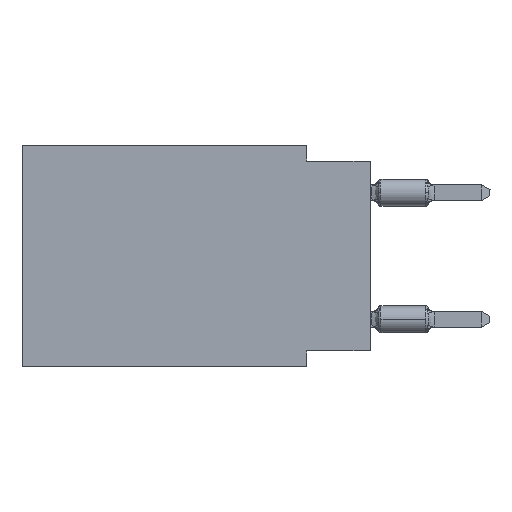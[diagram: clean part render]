
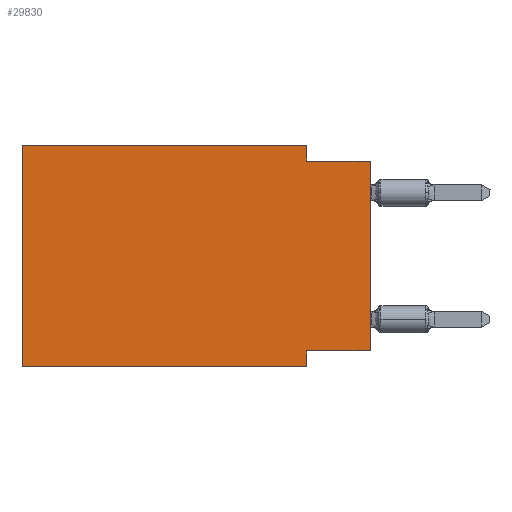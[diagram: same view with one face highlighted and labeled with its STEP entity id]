
A CAD part, left-side view. The second image highlights one B-rep face of the part: STEP entity #29830.
In plain terms, the highlighted planar face has unit normal (-1, 0, 0).
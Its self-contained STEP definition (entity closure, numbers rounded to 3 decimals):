
#336 = LINE ( 'NONE', #10719, #8481 ) ;
#1377 = DIRECTION ( 'NONE',  ( 0., 0., 1. ) ) ;
#1556 = VECTOR ( 'NONE', #22033, 1000. ) ;
#1713 = EDGE_CURVE ( 'NONE', #9683, #20176, #336, .T. ) ;
#1868 = PLANE ( 'NONE',  #12691 ) ;
#3215 = LINE ( 'NONE', #22807, #13539 ) ;
#3859 = CARTESIAN_POINT ( 'NONE',  ( 0., 0., 0. ) ) ;
#4535 = DIRECTION ( 'NONE',  ( 0., -1., 0. ) ) ;
#4771 = CARTESIAN_POINT ( 'NONE',  ( 0., 2.54, 0. ) ) ;
#5603 = VECTOR ( 'NONE', #4535, 1000. ) ;
#5838 = DIRECTION ( 'NONE',  ( 0., -1., 0. ) ) ;
#6252 = EDGE_CURVE ( 'NONE', #9683, #6913, #14470, .T. ) ;
#6913 = VERTEX_POINT ( 'NONE', #9599 ) ;
#7314 = DIRECTION ( 'NONE',  ( 0., 0., -1. ) ) ;
#7605 = VERTEX_POINT ( 'NONE', #26460 ) ;
#7999 = CARTESIAN_POINT ( 'NONE',  ( 0., 13.97, -8.89 ) ) ;
#8481 = VECTOR ( 'NONE', #11057, 1000. ) ;
#8502 = CARTESIAN_POINT ( 'NONE',  ( 0., 0., -0.635 ) ) ;
#8639 = CARTESIAN_POINT ( 'NONE',  ( 0., 0., -0.635 ) ) ;
#8803 = LINE ( 'NONE', #31326, #17737 ) ;
#9553 = EDGE_CURVE ( 'NONE', #20176, #31836, #17046, .T. ) ;
#9599 = CARTESIAN_POINT ( 'NONE',  ( 0., 2.54, -8.89 ) ) ;
#9612 = LINE ( 'NONE', #24917, #18871 ) ;
#9683 = VERTEX_POINT ( 'NONE', #7999 ) ;
#9808 = ORIENTED_EDGE ( 'NONE', *, *, #12927, .T. ) ;
#9941 = CARTESIAN_POINT ( 'NONE',  ( 0., 13.97, 0. ) ) ;
#10511 = EDGE_CURVE ( 'NONE', #31836, #32505, #8803, .T. ) ;
#10719 = CARTESIAN_POINT ( 'NONE',  ( 0., 13.97, 0. ) ) ;
#11057 = DIRECTION ( 'NONE',  ( 0., 0., 1. ) ) ;
#12691 = AXIS2_PLACEMENT_3D ( 'NONE', #9941, #27209, #7314 ) ;
#12927 = EDGE_CURVE ( 'NONE', #7605, #14145, #16376, .T. ) ;
#13094 = DIRECTION ( 'NONE',  ( 0., 1., 0. ) ) ;
#13539 = VECTOR ( 'NONE', #13094, 1000. ) ;
#13788 = VERTEX_POINT ( 'NONE', #15812 ) ;
#14119 = EDGE_CURVE ( 'NONE', #7605, #13788, #3215, .T. ) ;
#14145 = VERTEX_POINT ( 'NONE', #8502 ) ;
#14470 = LINE ( 'NONE', #24503, #1556 ) ;
#15230 = ORIENTED_EDGE ( 'NONE', *, *, #6252, .T. ) ;
#15557 = VECTOR ( 'NONE', #1377, 1000. ) ;
#15812 = CARTESIAN_POINT ( 'NONE',  ( 0., 2.54, -8.255 ) ) ;
#15906 = ORIENTED_EDGE ( 'NONE', *, *, #19904, .F. ) ;
#16048 = EDGE_CURVE ( 'NONE', #13788, #6913, #9612, .T. ) ;
#16376 = LINE ( 'NONE', #3859, #15557 ) ;
#16941 = ORIENTED_EDGE ( 'NONE', *, *, #9553, .F. ) ;
#17046 = LINE ( 'NONE', #32017, #5603 ) ;
#17557 = ORIENTED_EDGE ( 'NONE', *, *, #16048, .F. ) ;
#17737 = VECTOR ( 'NONE', #23283, 1000. ) ;
#17920 = ORIENTED_EDGE ( 'NONE', *, *, #1713, .F. ) ;
#18019 = ORIENTED_EDGE ( 'NONE', *, *, #14119, .F. ) ;
#18871 = VECTOR ( 'NONE', #19647, 1000. ) ;
#19647 = DIRECTION ( 'NONE',  ( 0., 0., -1. ) ) ;
#19904 = EDGE_CURVE ( 'NONE', #32505, #14145, #31003, .T. ) ;
#20148 = FACE_OUTER_BOUND ( 'NONE', #31575, .T. ) ;
#20176 = VERTEX_POINT ( 'NONE', #27845 ) ;
#22033 = DIRECTION ( 'NONE',  ( 0., -1., 0. ) ) ;
#22807 = CARTESIAN_POINT ( 'NONE',  ( 0., 0., -8.255 ) ) ;
#23283 = DIRECTION ( 'NONE',  ( 0., 0., -1. ) ) ;
#23754 = VECTOR ( 'NONE', #5838, 1000. ) ;
#24503 = CARTESIAN_POINT ( 'NONE',  ( 0., 13.97, -8.89 ) ) ;
#24917 = CARTESIAN_POINT ( 'NONE',  ( 0., 2.54, -8.89 ) ) ;
#26460 = CARTESIAN_POINT ( 'NONE',  ( 0., 0., -8.255 ) ) ;
#27209 = DIRECTION ( 'NONE',  ( 1., 0., 0. ) ) ;
#27845 = CARTESIAN_POINT ( 'NONE',  ( 0., 13.97, 0. ) ) ;
#28951 = ORIENTED_EDGE ( 'NONE', *, *, #10511, .F. ) ;
#29830 = ADVANCED_FACE ( 'NONE', ( #20148 ), #1868, .F. ) ;
#31003 = LINE ( 'NONE', #8639, #23754 ) ;
#31326 = CARTESIAN_POINT ( 'NONE',  ( 0., 2.54, 0. ) ) ;
#31575 = EDGE_LOOP ( 'NONE', ( #9808, #15906, #28951, #16941, #17920, #15230, #17557, #18019 ) ) ;
#31836 = VERTEX_POINT ( 'NONE', #4771 ) ;
#32017 = CARTESIAN_POINT ( 'NONE',  ( 0., 13.97, 0. ) ) ;
#32034 = CARTESIAN_POINT ( 'NONE',  ( 0., 2.54, -0.635 ) ) ;
#32505 = VERTEX_POINT ( 'NONE', #32034 ) ;
